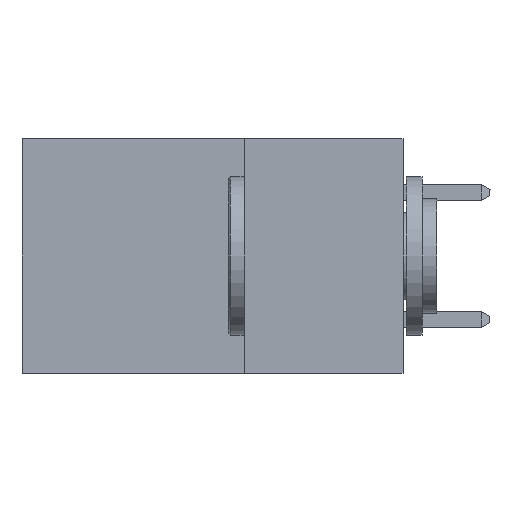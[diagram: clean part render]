
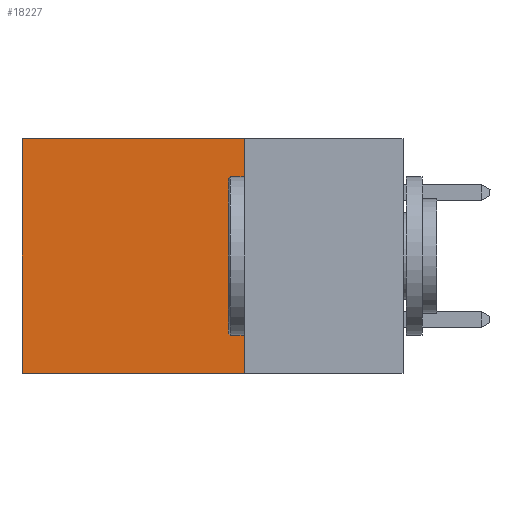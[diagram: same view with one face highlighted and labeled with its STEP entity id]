
A CAD part, left-side view. The second image highlights one B-rep face of the part: STEP entity #18227.
In plain terms, the highlighted planar face has unit normal (-1, 0, 0).
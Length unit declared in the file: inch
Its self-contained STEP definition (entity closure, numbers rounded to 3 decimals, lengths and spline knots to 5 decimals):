
#931 = EDGE_CURVE ( 'NONE', #6687, #6085, #6221, .T. ) ;
#1042 = DIRECTION ( 'NONE',  ( 0., 1., 0. ) ) ;
#1253 = PLANE ( 'NONE',  #7721 ) ;
#1283 = LINE ( 'NONE', #29411, #19284 ) ;
#2280 = VERTEX_POINT ( 'NONE', #24113 ) ;
#3528 = EDGE_CURVE ( 'NONE', #22694, #6085, #1283, .T. ) ;
#4657 = CARTESIAN_POINT ( 'NONE',  ( 0.2875, 0.6, 0. ) ) ;
#5828 = CARTESIAN_POINT ( 'NONE',  ( 0.2875, 0.25, -0.37 ) ) ;
#6085 = VERTEX_POINT ( 'NONE', #8295 ) ;
#6221 = LINE ( 'NONE', #22248, #12809 ) ;
#6687 = VERTEX_POINT ( 'NONE', #4657 ) ;
#7721 = AXIS2_PLACEMENT_3D ( 'NONE', #17695, #8327, #24828 ) ;
#8000 = CARTESIAN_POINT ( 'NONE',  ( 0.2875, 0.25, 0. ) ) ;
#8295 = CARTESIAN_POINT ( 'NONE',  ( 0.2875, 0.6, -0.37 ) ) ;
#8327 = DIRECTION ( 'NONE',  ( 1., 0., 0. ) ) ;
#9165 = EDGE_LOOP ( 'NONE', ( #25008, #24574, #10263, #24635 ) ) ;
#9777 = VECTOR ( 'NONE', #10190, 39.37008 ) ;
#9803 = EDGE_CURVE ( 'NONE', #2280, #22694, #19323, .T. ) ;
#10190 = DIRECTION ( 'NONE',  ( 0., 0., -1. ) ) ;
#10263 = ORIENTED_EDGE ( 'NONE', *, *, #9803, .F. ) ;
#12320 = LINE ( 'NONE', #8000, #29645 ) ;
#12809 = VECTOR ( 'NONE', #17827, 39.37008 ) ;
#13064 = FACE_OUTER_BOUND ( 'NONE', #9165, .T. ) ;
#17086 = EDGE_CURVE ( 'NONE', #2280, #6687, #12320, .T. ) ;
#17695 = CARTESIAN_POINT ( 'NONE',  ( 0.2875, 0.25, 0. ) ) ;
#17827 = DIRECTION ( 'NONE',  ( 0., 0., -1. ) ) ;
#18227 = ADVANCED_FACE ( 'NONE', ( #13064 ), #1253, .F. ) ;
#19284 = VECTOR ( 'NONE', #26633, 39.37008 ) ;
#19323 = LINE ( 'NONE', #27023, #9777 ) ;
#22248 = CARTESIAN_POINT ( 'NONE',  ( 0.2875, 0.6, 0. ) ) ;
#22694 = VERTEX_POINT ( 'NONE', #5828 ) ;
#24113 = CARTESIAN_POINT ( 'NONE',  ( 0.2875, 0.25, 0. ) ) ;
#24574 = ORIENTED_EDGE ( 'NONE', *, *, #3528, .F. ) ;
#24635 = ORIENTED_EDGE ( 'NONE', *, *, #17086, .T. ) ;
#24828 = DIRECTION ( 'NONE',  ( 0., 0., -1. ) ) ;
#25008 = ORIENTED_EDGE ( 'NONE', *, *, #931, .T. ) ;
#26633 = DIRECTION ( 'NONE',  ( 0., 1., 0. ) ) ;
#27023 = CARTESIAN_POINT ( 'NONE',  ( 0.2875, 0.25, 0. ) ) ;
#29411 = CARTESIAN_POINT ( 'NONE',  ( 0.2875, 0.25, -0.37 ) ) ;
#29645 = VECTOR ( 'NONE', #1042, 39.37008 ) ;
